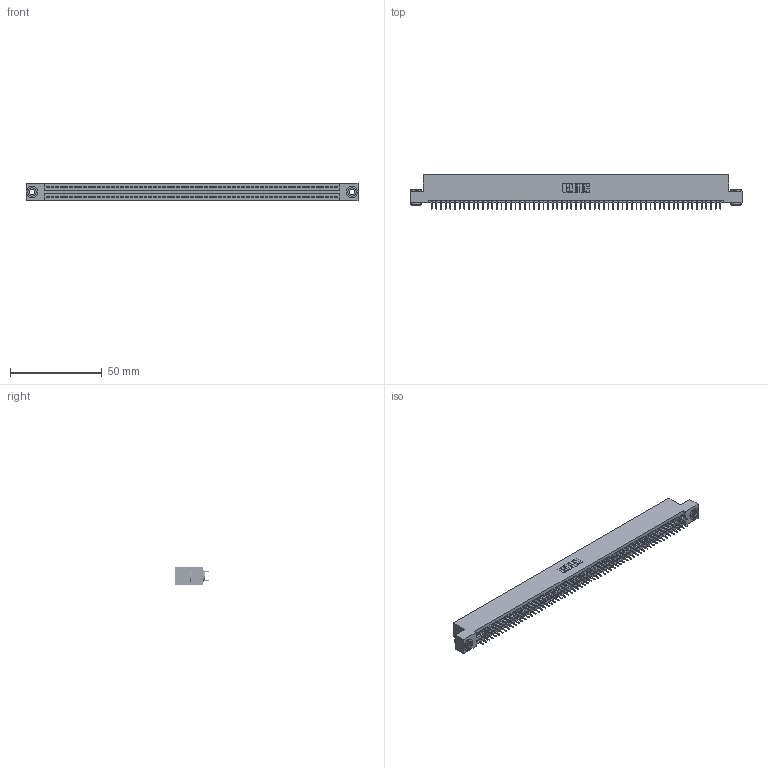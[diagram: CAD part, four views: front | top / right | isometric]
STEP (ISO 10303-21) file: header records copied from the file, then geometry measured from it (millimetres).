
FILE_DESCRIPTION (( 'STEP AP203' ), '1' );
FILE_NAME ('845-126-525-203.STEP', '2020-09-24T11:03:25', ( '' ), ( '' ), 'SwSTEP 2.0', 'SolidWorks 2020', '' );
FILE_SCHEMA (( 'CONFIG_CONTROL_DESIGN' ));
Length unit declared in the file: inch
Products named in the file (4): 845 Part_Flush Mounting Lugs - 0.156 Dia-TH; 845-126-525-203; 345-250-002_345-250-002-102; 345-292-001_345-293-125
Assembly tree (129 placements, depth 2):
  845-126-525-203
    845 Part_Flush Mounting Lugs - 0.156 Dia-TH
    345-292-001_345-293-125  x126
    345-250-002_345-250-002-102  x2
Bounding box: 181.23 x 18.72 x 9.4 mm (x, y, z)
Volume: 17611.7 mm3; surface area: 26019.7 mm2
Topology: 129 solids, 129 shells, 6968 faces, 19695 edges, 12622 vertices
Faces by surface type: plane 5004, cylinder 1956, cone 8
Entity records: 47328 total; most frequent: CARTESIAN_POINT 7887, ORIENTED_EDGE 7814, DIRECTION 6961, EDGE_CURVE 3907, VECTOR 3503, LINE 3503, VERTEX_POINT 2598, AXIS2_PLACEMENT_3D 1729
